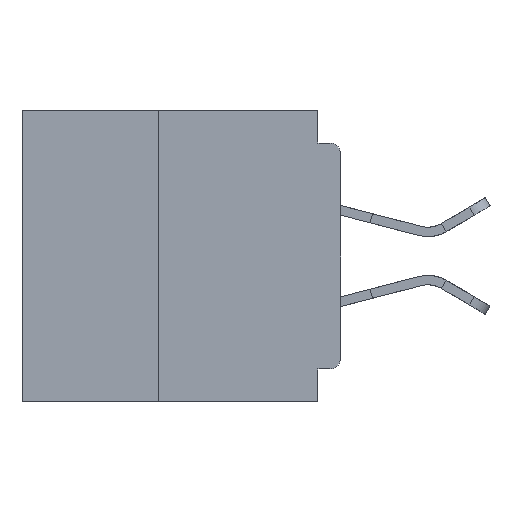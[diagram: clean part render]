
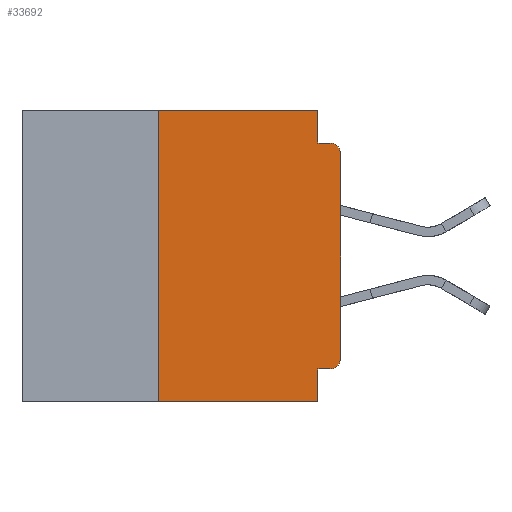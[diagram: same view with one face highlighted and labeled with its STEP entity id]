
A CAD part, left-side view. The second image highlights one B-rep face of the part: STEP entity #33692.
In plain terms, the highlighted planar face has unit normal (-1, 0, 0).
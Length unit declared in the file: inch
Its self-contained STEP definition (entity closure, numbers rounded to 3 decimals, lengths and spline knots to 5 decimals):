
#239 = LINE ( 'NONE', #6706, #19563 ) ;
#715 = LINE ( 'NONE', #12324, #24498 ) ;
#765 = DIRECTION ( 'NONE',  ( 0., 0., -1. ) ) ;
#1827 = EDGE_CURVE ( 'NONE', #17044, #25934, #38677, .T. ) ;
#2071 = VECTOR ( 'NONE', #26221, 39.37008 ) ;
#2363 = CARTESIAN_POINT ( 'NONE',  ( 0., 0.031, -0.4 ) ) ;
#2922 = EDGE_CURVE ( 'NONE', #16492, #25614, #239, .T. ) ;
#3120 = LINE ( 'NONE', #32747, #2071 ) ;
#3182 = ORIENTED_EDGE ( 'NONE', *, *, #32481, .F. ) ;
#3994 = CARTESIAN_POINT ( 'NONE',  ( 0., 0., 0. ) ) ;
#5129 = EDGE_CURVE ( 'NONE', #25270, #6899, #7758, .T. ) ;
#6359 = CARTESIAN_POINT ( 'NONE',  ( 0., 0., -0.34 ) ) ;
#6706 = CARTESIAN_POINT ( 'NONE',  ( 0., 0.25, -0.4 ) ) ;
#6893 = ORIENTED_EDGE ( 'NONE', *, *, #10659, .F. ) ;
#6899 = VERTEX_POINT ( 'NONE', #29348 ) ;
#7570 = LINE ( 'NONE', #40843, #8628 ) ;
#7758 = LINE ( 'NONE', #14202, #23820 ) ;
#7803 = CARTESIAN_POINT ( 'NONE',  ( 0., 0.015, -0.355 ) ) ;
#8628 = VECTOR ( 'NONE', #21738, 39.37008 ) ;
#9066 = ORIENTED_EDGE ( 'NONE', *, *, #2922, .F. ) ;
#9109 = DIRECTION ( 'NONE',  ( 0., 1., 0. ) ) ;
#10018 = LINE ( 'NONE', #39366, #25987 ) ;
#10432 = VECTOR ( 'NONE', #33033, 39.37008 ) ;
#10659 = EDGE_CURVE ( 'NONE', #35087, #29689, #16838, .T. ) ;
#10943 = CARTESIAN_POINT ( 'NONE',  ( 0., 0.015, -0.34 ) ) ;
#11279 = ORIENTED_EDGE ( 'NONE', *, *, #36078, .T. ) ;
#11542 = FACE_OUTER_BOUND ( 'NONE', #38320, .T. ) ;
#12324 = CARTESIAN_POINT ( 'NONE',  ( 0., 0., -0.045 ) ) ;
#12466 = DIRECTION ( 'NONE',  ( 0., -1., 0. ) ) ;
#12573 = PLANE ( 'NONE',  #23663 ) ;
#13056 = ORIENTED_EDGE ( 'NONE', *, *, #5129, .F. ) ;
#13629 = AXIS2_PLACEMENT_3D ( 'NONE', #10943, #33363, #14185 ) ;
#14185 = DIRECTION ( 'NONE',  ( 0., 0., -1. ) ) ;
#14202 = CARTESIAN_POINT ( 'NONE',  ( 0., 0.031, 0. ) ) ;
#14370 = CARTESIAN_POINT ( 'NONE',  ( 0., 0.015, -0.06 ) ) ;
#15826 = DIRECTION ( 'NONE',  ( 1., 0., 0. ) ) ;
#16350 = DIRECTION ( 'NONE',  ( 0., 0., 1. ) ) ;
#16492 = VERTEX_POINT ( 'NONE', #33868 ) ;
#16838 = LINE ( 'NONE', #37925, #41268 ) ;
#17044 = VERTEX_POINT ( 'NONE', #40447 ) ;
#17315 = ORIENTED_EDGE ( 'NONE', *, *, #25641, .F. ) ;
#17424 = DIRECTION ( 'NONE',  ( 0., 0., -1. ) ) ;
#18189 = DIRECTION ( 'NONE',  ( -1., 0., 0. ) ) ;
#19563 = VECTOR ( 'NONE', #16350, 39.37008 ) ;
#19984 = DIRECTION ( 'NONE',  ( 0., 0., -1. ) ) ;
#20114 = CARTESIAN_POINT ( 'NONE',  ( 0., 0.015, -0.045 ) ) ;
#21738 = DIRECTION ( 'NONE',  ( 0., -1., 0. ) ) ;
#22007 = ORIENTED_EDGE ( 'NONE', *, *, #33977, .F. ) ;
#22140 = AXIS2_PLACEMENT_3D ( 'NONE', #14370, #18189, #19984 ) ;
#22981 = VERTEX_POINT ( 'NONE', #2363 ) ;
#23663 = AXIS2_PLACEMENT_3D ( 'NONE', #34956, #15826, #38136 ) ;
#23820 = VECTOR ( 'NONE', #17424, 39.37008 ) ;
#24498 = VECTOR ( 'NONE', #12466, 39.37008 ) ;
#25270 = VERTEX_POINT ( 'NONE', #39175 ) ;
#25614 = VERTEX_POINT ( 'NONE', #40921 ) ;
#25641 = EDGE_CURVE ( 'NONE', #6899, #25934, #715, .T. ) ;
#25934 = VERTEX_POINT ( 'NONE', #20114 ) ;
#25987 = VECTOR ( 'NONE', #765, 39.37008 ) ;
#26221 = DIRECTION ( 'NONE',  ( 0., -1., 0. ) ) ;
#28101 = ORIENTED_EDGE ( 'NONE', *, *, #35066, .T. ) ;
#29348 = CARTESIAN_POINT ( 'NONE',  ( 0., 0.031, -0.045 ) ) ;
#29689 = VERTEX_POINT ( 'NONE', #32710 ) ;
#30151 = VERTEX_POINT ( 'NONE', #6359 ) ;
#32481 = EDGE_CURVE ( 'NONE', #25614, #25270, #7570, .T. ) ;
#32710 = CARTESIAN_POINT ( 'NONE',  ( 0., 0.031, -0.355 ) ) ;
#32747 = CARTESIAN_POINT ( 'NONE',  ( 0., 0.437, -0.4 ) ) ;
#33033 = DIRECTION ( 'NONE',  ( 0., 0., 1. ) ) ;
#33363 = DIRECTION ( 'NONE',  ( -1., 0., 0. ) ) ;
#33692 = ADVANCED_FACE ( 'NONE', ( #11542 ), #12573, .F. ) ;
#33868 = CARTESIAN_POINT ( 'NONE',  ( 0., 0.25, -0.4 ) ) ;
#33971 = CIRCLE ( 'NONE', #13629, 0.015 ) ;
#33977 = EDGE_CURVE ( 'NONE', #29689, #22981, #10018, .T. ) ;
#34956 = CARTESIAN_POINT ( 'NONE',  ( 0., 0.437, 0. ) ) ;
#35066 = EDGE_CURVE ( 'NONE', #35087, #30151, #33971, .T. ) ;
#35087 = VERTEX_POINT ( 'NONE', #7803 ) ;
#35951 = LINE ( 'NONE', #3994, #10432 ) ;
#36078 = EDGE_CURVE ( 'NONE', #16492, #22981, #3120, .T. ) ;
#37925 = CARTESIAN_POINT ( 'NONE',  ( 0., 0., -0.355 ) ) ;
#38136 = DIRECTION ( 'NONE',  ( 0., 0., -1. ) ) ;
#38320 = EDGE_LOOP ( 'NONE', ( #40294, #38838, #17315, #13056, #3182, #9066, #11279, #22007, #6893, #28101 ) ) ;
#38528 = EDGE_CURVE ( 'NONE', #30151, #17044, #35951, .T. ) ;
#38677 = CIRCLE ( 'NONE', #22140, 0.015 ) ;
#38838 = ORIENTED_EDGE ( 'NONE', *, *, #1827, .T. ) ;
#39175 = CARTESIAN_POINT ( 'NONE',  ( 0., 0.031, 0. ) ) ;
#39366 = CARTESIAN_POINT ( 'NONE',  ( 0., 0.031, -0.4 ) ) ;
#40294 = ORIENTED_EDGE ( 'NONE', *, *, #38528, .T. ) ;
#40447 = CARTESIAN_POINT ( 'NONE',  ( 0., 0., -0.06 ) ) ;
#40843 = CARTESIAN_POINT ( 'NONE',  ( 0., 0.437, 0. ) ) ;
#40921 = CARTESIAN_POINT ( 'NONE',  ( 0., 0.25, 0. ) ) ;
#41268 = VECTOR ( 'NONE', #9109, 39.37008 ) ;
